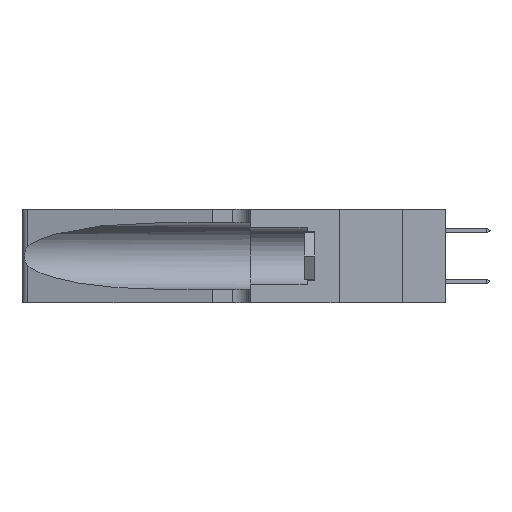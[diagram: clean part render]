
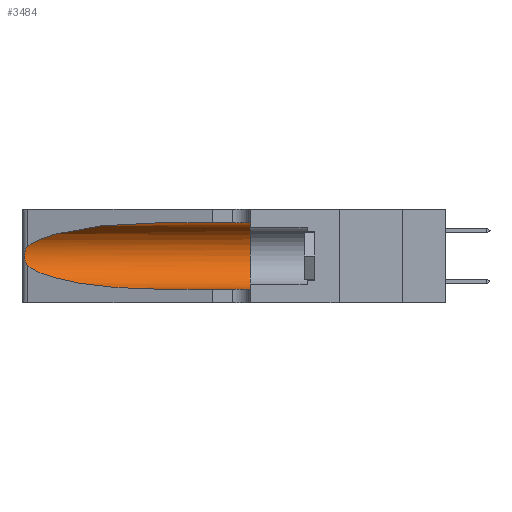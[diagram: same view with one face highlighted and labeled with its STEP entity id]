
A CAD part, left-side view. The second image highlights one B-rep face of the part: STEP entity #3484.
In plain terms, the highlighted cylindrical face has radius 3.308 mm (diameter 6.617 mm), a partial arc.
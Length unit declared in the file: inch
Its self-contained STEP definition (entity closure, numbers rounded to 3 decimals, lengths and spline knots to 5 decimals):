
#130 = VERTEX_POINT ( 'NONE', #5156 ) ;
#818 = CARTESIAN_POINT ( 'NONE',  ( 0.25555, 1.22994, 0.2215 ) ) ;
#847 = VERTEX_POINT ( 'NONE', #3210 ) ;
#976 = VERTEX_POINT ( 'NONE', #18008 ) ;
#1526 = EDGE_LOOP ( 'NONE', ( #27182, #26638, #21966, #11000, #7488, #28772 ) ) ;
#2366 = AXIS2_PLACEMENT_3D ( 'NONE', #24455, #11071, #16341 ) ;
#2568 = DIRECTION ( 'NONE',  ( 0., 0., -1. ) ) ;
#2782 = CARTESIAN_POINT ( 'NONE',  ( 0.25487, 1.22718, 0.22369 ) ) ;
#2881 = CARTESIAN_POINT ( 'NONE',  ( 0.1305, 0.72297, 0.05475 ) ) ;
#3186 = CARTESIAN_POINT ( 'NONE',  ( 0.1305, 1.61858, 0.05475 ) ) ;
#3210 = CARTESIAN_POINT ( 'NONE',  ( 0.1305, 0.72297, 0.31525 ) ) ;
#3307 = CARTESIAN_POINT ( 'NONE',  ( 0.25789, 1.23486, 0.15765 ) ) ;
#3484 = ADVANCED_FACE ( 'NONE', ( #8337 ), #11353, .F. ) ;
#4100 = LINE ( 'NONE', #3186, #21588 ) ;
#4170 = CARTESIAN_POINT ( 'NONE',  ( 0.26075, 1.23896, 0.178 ) ) ;
#4894 = CARTESIAN_POINT ( 'NONE',  ( 0.2373, 1.15595, 0.08982 ) ) ;
#5156 = CARTESIAN_POINT ( 'NONE',  ( 0.25487, 1.22718, 0.14631 ) ) ;
#6292 = CARTESIAN_POINT ( 'NONE',  ( 0.25639, 1.23186, 0.15144 ) ) ;
#6386 = VERTEX_POINT ( 'NONE', #28887 ) ;
#6551 = LINE ( 'NONE', #30033, #15494 ) ;
#6949 = EDGE_CURVE ( 'NONE', #6386, #130, #29302, .T. ) ;
#7488 = ORIENTED_EDGE ( 'NONE', *, *, #22183, .F. ) ;
#7852 = CARTESIAN_POINT ( 'NONE',  ( 0.26017, 1.23833, 0.17102 ) ) ;
#8337 = FACE_OUTER_BOUND ( 'NONE', #1526, .T. ) ;
#9202 = CARTESIAN_POINT ( 'NONE',  ( 0.25639, 1.23184, 0.21858 ) ) ;
#9681 = CARTESIAN_POINT ( 'NONE',  ( 0.25854, 1.2359, 0.20912 ) ) ;
#11000 = ORIENTED_EDGE ( 'NONE', *, *, #22395, .T. ) ;
#11071 = DIRECTION ( 'NONE',  ( 0., 1., 0. ) ) ;
#11353 = CYLINDRICAL_SURFACE ( 'NONE', #32149, 0.13025 ) ;
#13405 = VERTEX_POINT ( 'NONE', #2881 ) ;
#13510 = CIRCLE ( 'NONE', #2366, 0.13025 ) ;
#13996 =( BOUNDED_CURVE ( )  B_SPLINE_CURVE ( 3, ( #27743, #16297, #27276, #2782 ),
 .UNSPECIFIED., .F., .F. ) 
 B_SPLINE_CURVE_WITH_KNOTS ( ( 4, 4 ),
 ( 1.5708, 2.84003 ),
 .UNSPECIFIED. ) 
 CURVE ( )  GEOMETRIC_REPRESENTATION_ITEM ( )  RATIONAL_B_SPLINE_CURVE ( ( 1., 0.87, 0.87, 1. ) ) 
 REPRESENTATION_ITEM ( '' )  );
#14519 = CARTESIAN_POINT ( 'NONE',  ( 0.25487, 1.22718, 0.14631 ) ) ;
#15494 = VECTOR ( 'NONE', #32553, 39.37008 ) ;
#15923 = VERTEX_POINT ( 'NONE', #26124 ) ;
#16297 = CARTESIAN_POINT ( 'NONE',  ( 0.18966, 0.96281, 0.31525 ) ) ;
#16341 = DIRECTION ( 'NONE',  ( 0., 0., 1. ) ) ;
#16689 = CARTESIAN_POINT ( 'NONE',  ( 0.25555, 1.22993, 0.14849 ) ) ;
#18008 = CARTESIAN_POINT ( 'NONE',  ( 0.1305, 0.35, 0.31525 ) ) ;
#18172 = CARTESIAN_POINT ( 'NONE',  ( 0.26018, 1.23835, 0.19895 ) ) ;
#20983 = CARTESIAN_POINT ( 'NONE',  ( 0.25856, 1.23593, 0.16098 ) ) ;
#21588 = VECTOR ( 'NONE', #25147, 39.37008 ) ;
#21605 = CARTESIAN_POINT ( 'NONE',  ( 0.1305, 0.72297, 0.05475 ) ) ;
#21966 = ORIENTED_EDGE ( 'NONE', *, *, #27428, .T. ) ;
#22183 = EDGE_CURVE ( 'NONE', #976, #15923, #13510, .T. ) ;
#22395 = EDGE_CURVE ( 'NONE', #13405, #15923, #4100, .T. ) ;
#22580 = CARTESIAN_POINT ( 'NONE',  ( 0.25787, 1.23484, 0.2124 ) ) ;
#24455 = CARTESIAN_POINT ( 'NONE',  ( 0.1305, 0.35, 0.185 ) ) ;
#25010 = EDGE_CURVE ( 'NONE', #847, #6386, #13996, .T. ) ;
#25147 = DIRECTION ( 'NONE',  ( 0., -1., 0. ) ) ;
#25798 = CARTESIAN_POINT ( 'NONE',  ( 0.25487, 1.22718, 0.22369 ) ) ;
#26124 = CARTESIAN_POINT ( 'NONE',  ( 0.1305, 0.35, 0.05475 ) ) ;
#26162 = EDGE_CURVE ( 'NONE', #847, #976, #6551, .T. ) ;
#26638 = ORIENTED_EDGE ( 'NONE', *, *, #6949, .T. ) ;
#27073 = DIRECTION ( 'NONE',  ( 0., -1., 0. ) ) ;
#27182 = ORIENTED_EDGE ( 'NONE', *, *, #25010, .T. ) ;
#27276 = CARTESIAN_POINT ( 'NONE',  ( 0.2373, 1.15595, 0.28018 ) ) ;
#27428 = EDGE_CURVE ( 'NONE', #130, #13405, #35202, .T. ) ;
#27743 = CARTESIAN_POINT ( 'NONE',  ( 0.1305, 0.72297, 0.31525 ) ) ;
#28635 = CARTESIAN_POINT ( 'NONE',  ( 0.26075, 1.23896, 0.19203 ) ) ;
#28772 = ORIENTED_EDGE ( 'NONE', *, *, #26162, .F. ) ;
#28887 = CARTESIAN_POINT ( 'NONE',  ( 0.25487, 1.22718, 0.22369 ) ) ;
#29302 = B_SPLINE_CURVE_WITH_KNOTS ( 'NONE', 3,
 ( #25798, #818, #9202, #22580, #9681, #18172, #28635, #4170, #7852, #20983, #3307, #6292, #16689, #14519 ),
 .UNSPECIFIED., .F., .F.,
 ( 4, 2, 2, 2, 2, 2, 4 ),
 ( 0., 0.00027, 0.00053, 0.00107, 0.0016, 0.00187, 0.00214 ),
 .UNSPECIFIED. ) ;
#30033 = CARTESIAN_POINT ( 'NONE',  ( 0.1305, 1.61858, 0.31525 ) ) ;
#31988 = CARTESIAN_POINT ( 'NONE',  ( 0.1305, 1.61858, 0.185 ) ) ;
#32115 = CARTESIAN_POINT ( 'NONE',  ( 0.18966, 0.96281, 0.05475 ) ) ;
#32149 = AXIS2_PLACEMENT_3D ( 'NONE', #31988, #27073, #2568 ) ;
#32468 = CARTESIAN_POINT ( 'NONE',  ( 0.25487, 1.22718, 0.14631 ) ) ;
#32553 = DIRECTION ( 'NONE',  ( 0., -1., 0. ) ) ;
#35202 =( BOUNDED_CURVE ( )  B_SPLINE_CURVE ( 3, ( #32468, #4894, #32115, #21605 ),
 .UNSPECIFIED., .F., .F. ) 
 B_SPLINE_CURVE_WITH_KNOTS ( ( 4, 4 ),
 ( 3.44316, 4.71239 ),
 .UNSPECIFIED. ) 
 CURVE ( )  GEOMETRIC_REPRESENTATION_ITEM ( )  RATIONAL_B_SPLINE_CURVE ( ( 1., 0.87, 0.87, 1. ) ) 
 REPRESENTATION_ITEM ( '' )  );
